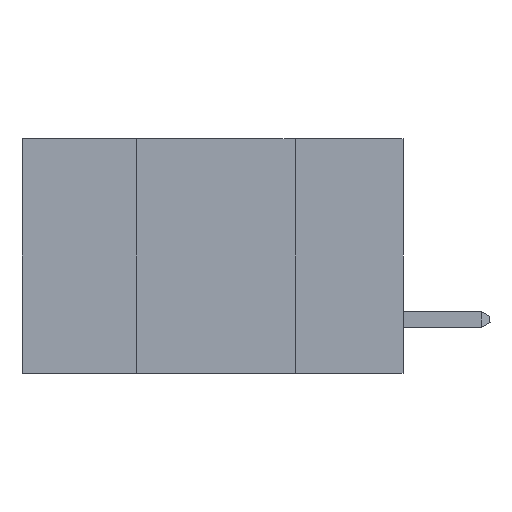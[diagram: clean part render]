
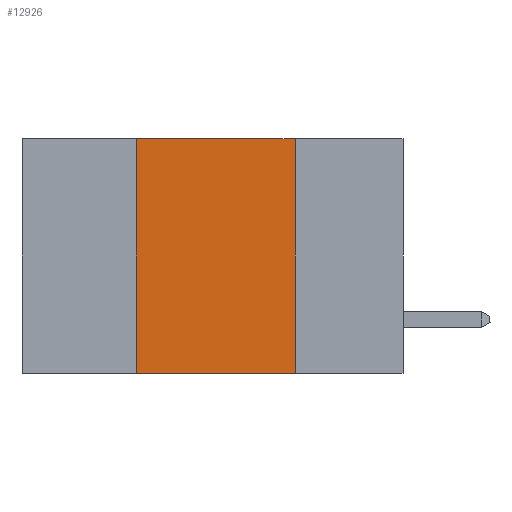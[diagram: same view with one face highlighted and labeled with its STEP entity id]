
A CAD part, left-side view. The second image highlights one B-rep face of the part: STEP entity #12926.
In plain terms, the highlighted planar face has unit normal (-1, 0, 0).
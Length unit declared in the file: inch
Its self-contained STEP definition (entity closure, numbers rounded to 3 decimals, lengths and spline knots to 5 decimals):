
#397 = CARTESIAN_POINT ( 'NONE',  ( 0., 0.42, 0. ) ) ;
#542 = CARTESIAN_POINT ( 'NONE',  ( 0., 0.42, 0. ) ) ;
#1020 = DIRECTION ( 'NONE',  ( 0., 0., -1. ) ) ;
#1780 = CARTESIAN_POINT ( 'NONE',  ( 0., 0.6, 0. ) ) ;
#2291 = DIRECTION ( 'NONE',  ( 0., -1., 0. ) ) ;
#2713 = VERTEX_POINT ( 'NONE', #26219 ) ;
#3301 = LINE ( 'NONE', #20386, #19868 ) ;
#3667 = DIRECTION ( 'NONE',  ( 0., 0., -1. ) ) ;
#3914 = EDGE_CURVE ( 'NONE', #2713, #6958, #18425, .T. ) ;
#4686 = ORIENTED_EDGE ( 'NONE', *, *, #3914, .F. ) ;
#5735 = EDGE_CURVE ( 'NONE', #2713, #22175, #20339, .T. ) ;
#6042 = PLANE ( 'NONE',  #26540 ) ;
#6958 = VERTEX_POINT ( 'NONE', #397 ) ;
#8127 = DIRECTION ( 'NONE',  ( 1., 0., 0. ) ) ;
#11297 = CARTESIAN_POINT ( 'NONE',  ( 0., 0.6, 0. ) ) ;
#12707 = VECTOR ( 'NONE', #2291, 39.37008 ) ;
#12926 = ADVANCED_FACE ( 'NONE', ( #18359 ), #6042, .F. ) ;
#13240 = DIRECTION ( 'NONE',  ( 0., 0., 1. ) ) ;
#14621 = VECTOR ( 'NONE', #19289, 39.37008 ) ;
#15452 = CARTESIAN_POINT ( 'NONE',  ( 0., 0.17, -0.37 ) ) ;
#16190 = VERTEX_POINT ( 'NONE', #19999 ) ;
#18359 = FACE_OUTER_BOUND ( 'NONE', #20924, .T. ) ;
#18421 = EDGE_CURVE ( 'NONE', #16190, #22175, #3301, .T. ) ;
#18425 = LINE ( 'NONE', #542, #27545 ) ;
#19289 = DIRECTION ( 'NONE',  ( 0., -1., 0. ) ) ;
#19453 = ORIENTED_EDGE ( 'NONE', *, *, #5735, .T. ) ;
#19868 = VECTOR ( 'NONE', #1020, 39.37008 ) ;
#19999 = CARTESIAN_POINT ( 'NONE',  ( 0., 0.17, 0. ) ) ;
#20339 = LINE ( 'NONE', #23811, #14621 ) ;
#20386 = CARTESIAN_POINT ( 'NONE',  ( 0., 0.17, 0. ) ) ;
#20924 = EDGE_LOOP ( 'NONE', ( #22448, #27613, #4686, #19453 ) ) ;
#20995 = EDGE_CURVE ( 'NONE', #6958, #16190, #27207, .T. ) ;
#22175 = VERTEX_POINT ( 'NONE', #15452 ) ;
#22448 = ORIENTED_EDGE ( 'NONE', *, *, #18421, .F. ) ;
#23811 = CARTESIAN_POINT ( 'NONE',  ( 0., 0.6, -0.37 ) ) ;
#26219 = CARTESIAN_POINT ( 'NONE',  ( 0., 0.42, -0.37 ) ) ;
#26540 = AXIS2_PLACEMENT_3D ( 'NONE', #1780, #8127, #3667 ) ;
#27207 = LINE ( 'NONE', #11297, #12707 ) ;
#27545 = VECTOR ( 'NONE', #13240, 39.37008 ) ;
#27613 = ORIENTED_EDGE ( 'NONE', *, *, #20995, .F. ) ;
